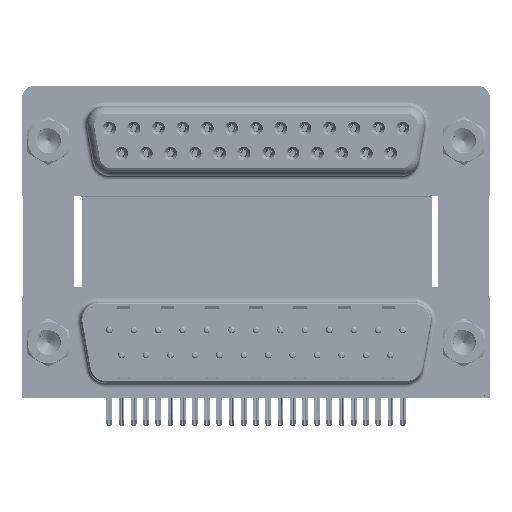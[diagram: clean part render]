
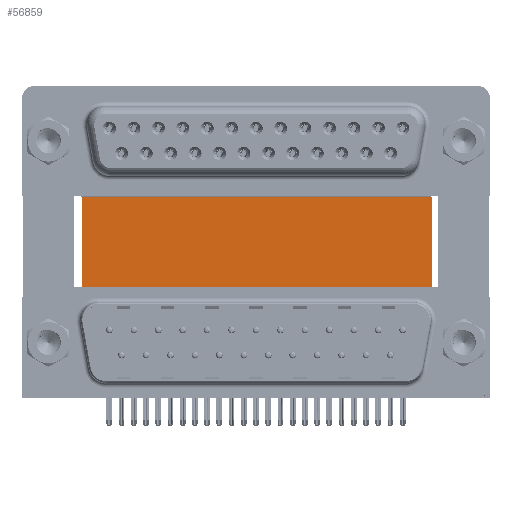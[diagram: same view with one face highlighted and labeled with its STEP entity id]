
A CAD part, top view. The second image highlights one B-rep face of the part: STEP entity #56859.
In plain terms, the highlighted planar face has unit normal (0, 0, 1).
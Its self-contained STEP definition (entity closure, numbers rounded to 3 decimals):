
#797 = CARTESIAN_POINT ( 'NONE',  ( 43.43, 16.585, -12. ) ) ;
#2367 = ORIENTED_EDGE ( 'NONE', *, *, #33299, .F. ) ;
#4066 = ORIENTED_EDGE ( 'NONE', *, *, #7551, .F. ) ;
#5335 = LINE ( 'NONE', #23770, #48347 ) ;
#7544 = DIRECTION ( 'NONE',  ( 0., 0., -1. ) ) ;
#7551 = EDGE_CURVE ( 'NONE', #46490, #18377, #44012, .T. ) ;
#13600 = LINE ( 'NONE', #797, #15337 ) ;
#13864 = EDGE_CURVE ( 'NONE', #25605, #43713, #15980, .T. ) ;
#15337 = VECTOR ( 'NONE', #42185, 1000. ) ;
#15980 = LINE ( 'NONE', #28994, #22403 ) ;
#16093 = AXIS2_PLACEMENT_3D ( 'NONE', #53478, #7544, #57691 ) ;
#17370 = CARTESIAN_POINT ( 'NONE',  ( 3.79, -3.735, -12. ) ) ;
#18377 = VERTEX_POINT ( 'NONE', #59347 ) ;
#19263 = DIRECTION ( 'NONE',  ( 0., -1., 0. ) ) ;
#21069 = ORIENTED_EDGE ( 'NONE', *, *, #37438, .T. ) ;
#22403 = VECTOR ( 'NONE', #47388, 1000. ) ;
#23770 = CARTESIAN_POINT ( 'NONE',  ( 3.79, 16.585, -12. ) ) ;
#25605 = VERTEX_POINT ( 'NONE', #17370 ) ;
#28994 = CARTESIAN_POINT ( 'NONE',  ( 3.79, -3.735, -12. ) ) ;
#33299 = EDGE_CURVE ( 'NONE', #18377, #43713, #13600, .T. ) ;
#33386 = EDGE_LOOP ( 'NONE', ( #37698, #2367, #4066, #21069 ) ) ;
#37438 = EDGE_CURVE ( 'NONE', #46490, #25605, #5335, .T. ) ;
#37698 = ORIENTED_EDGE ( 'NONE', *, *, #13864, .T. ) ;
#39273 = FACE_OUTER_BOUND ( 'NONE', #33386, .T. ) ;
#39498 = DIRECTION ( 'NONE',  ( 1., 0., 0. ) ) ;
#42185 = DIRECTION ( 'NONE',  ( 0., -1., 0. ) ) ;
#43713 = VERTEX_POINT ( 'NONE', #44596 ) ;
#44012 = LINE ( 'NONE', #57316, #51407 ) ;
#44596 = CARTESIAN_POINT ( 'NONE',  ( 43.43, -3.735, -12. ) ) ;
#46490 = VERTEX_POINT ( 'NONE', #50014 ) ;
#47388 = DIRECTION ( 'NONE',  ( 1., 0., 0. ) ) ;
#48347 = VECTOR ( 'NONE', #19263, 1000. ) ;
#50014 = CARTESIAN_POINT ( 'NONE',  ( 3.79, 16.585, -12. ) ) ;
#51407 = VECTOR ( 'NONE', #39498, 1000. ) ;
#52577 = PLANE ( 'NONE',  #16093 ) ;
#53478 = CARTESIAN_POINT ( 'NONE',  ( 3.79, 16.585, -12. ) ) ;
#56859 = ADVANCED_FACE ( 'NONE', ( #39273 ), #52577, .F. ) ;
#57316 = CARTESIAN_POINT ( 'NONE',  ( 3.79, 16.585, -12. ) ) ;
#57691 = DIRECTION ( 'NONE',  ( -1., 0., 0. ) ) ;
#59347 = CARTESIAN_POINT ( 'NONE',  ( 43.43, 16.585, -12. ) ) ;
